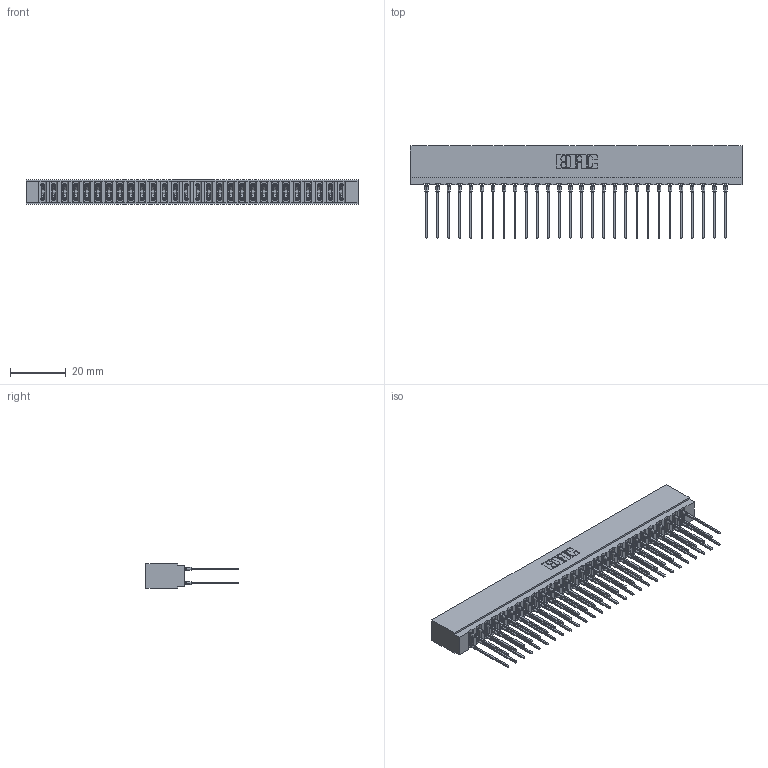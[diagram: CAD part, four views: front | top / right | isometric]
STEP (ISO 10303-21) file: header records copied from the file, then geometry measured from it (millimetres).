
FILE_DESCRIPTION (( 'STEP AP203' ), '1' );
FILE_NAME ('717-056-541-201.STEP', '2026-02-20T18:28:35', ( '' ), ( '' ), 'SwSTEP 2.0', 'SolidWorks 2023', '' );
FILE_SCHEMA (( 'CONFIG_CONTROL_DESIGN' ));
Length unit declared in the file: millimetre
Products named in the file (3): 717 Part_Insulator Option - 06; 717-056-541-201; 745-292-001_541
Assembly tree (57 placements, depth 2):
  717-056-541-201
    717 Part_Insulator Option - 06
    745-292-001_541  x56
Bounding box: 118.82 x 33.01 x 8.89 mm (x, y, z)
Volume: 10627.9 mm3; surface area: 17317.3 mm2
Topology: 57 solids, 57 shells, 5134 faces, 13803 edges, 8678 vertices
Faces by surface type: plane 2658, bspline 1120, cylinder 1020, torus 336
Entity records: 49905 total; most frequent: CARTESIAN_POINT 9169, ORIENTED_EDGE 8576, DIRECTION 7500, EDGE_CURVE 4288, LINE 3938, VECTOR 3938, VERTEX_POINT 2738, AXIS2_PLACEMENT_3D 1781
